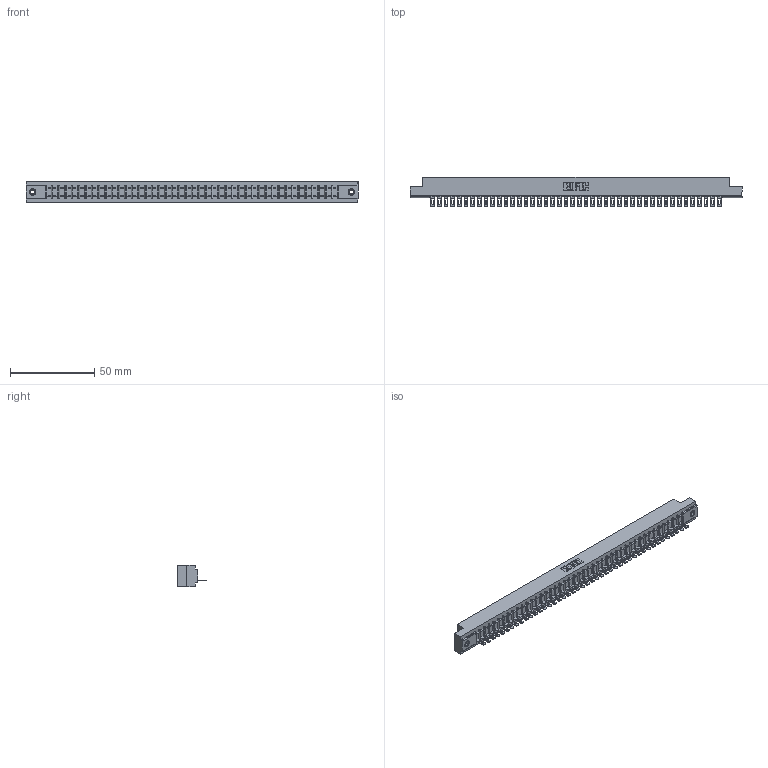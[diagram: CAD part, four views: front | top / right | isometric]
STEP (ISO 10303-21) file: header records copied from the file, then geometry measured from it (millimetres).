
FILE_DESCRIPTION (( 'STEP AP203' ), '1' );
FILE_NAME ('307-044-501-108.STEP', '2019-09-05T12:45:43', ( '' ), ( '' ), 'SwSTEP 2.0', 'SolidWorks 2016', '' );
FILE_SCHEMA (( 'CONFIG_CONTROL_DESIGN' ));
Length unit declared in the file: inch
Products named in the file (4): 345-250-001_345-250-003-102; 307-290-002_501; 307 Part_.156 Dia Mounting Holes; 307-044-501-108
Assembly tree (47 placements, depth 2):
  307-044-501-108
    307 Part_.156 Dia Mounting Holes
    307-290-002_501  x44
    345-250-001_345-250-003-102  x2
Bounding box: 197.36 x 17.42 x 12.7 mm (x, y, z)
Volume: 21166.5 mm3; surface area: 26974.4 mm2
Topology: 47 solids, 47 shells, 3567 faces, 10931 edges, 7158 vertices
Faces by surface type: plane 2038, cylinder 1423, sphere 90, cone 12, torus 4
Entity records: 39453 total; most frequent: CARTESIAN_POINT 6635, ORIENTED_EDGE 6618, DIRECTION 6459, EDGE_CURVE 3309, VECTOR 2531, LINE 2531, VERTEX_POINT 2140, AXIS2_PLACEMENT_3D 1964
